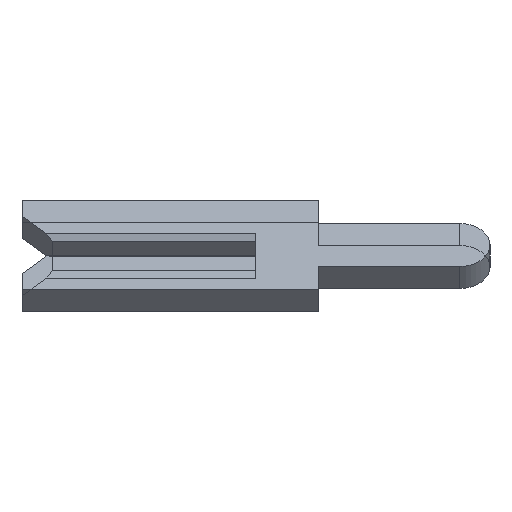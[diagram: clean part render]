
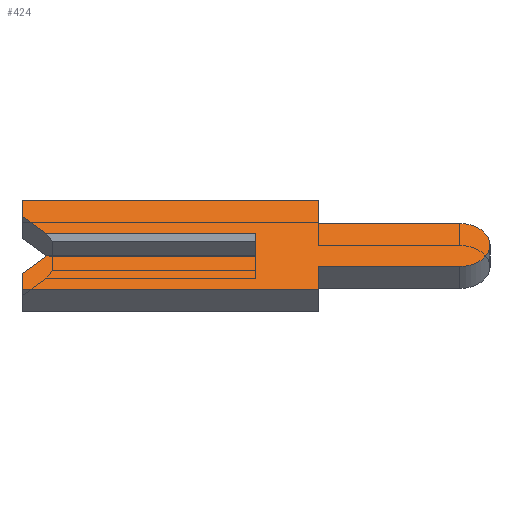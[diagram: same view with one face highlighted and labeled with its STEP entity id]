
A CAD part, left-side view. The second image highlights one B-rep face of the part: STEP entity #424.
In plain terms, the highlighted face is planar.
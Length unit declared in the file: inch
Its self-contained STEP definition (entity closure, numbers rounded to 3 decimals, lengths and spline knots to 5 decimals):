
#23 = CARTESIAN_POINT ( 'NONE',  ( -0.01, 0.15, -0.04 ) ) ;
#83 = EDGE_CURVE ( 'NONE', #255, #358, #2356, .T. ) ;
#101 = DIRECTION ( 'NONE',  ( 0., -0.707, 0.707 ) ) ;
#140 = CARTESIAN_POINT ( 'NONE',  ( -0.01, 0.15, 0.026 ) ) ;
#164 = ORIENTED_EDGE ( 'NONE', *, *, #291, .F. ) ;
#168 = VERTEX_POINT ( 'NONE', #1478 ) ;
#182 = CARTESIAN_POINT ( 'NONE',  ( -0.01, -0.1305, 0. ) ) ;
#186 = ORIENTED_EDGE ( 'NONE', *, *, #1485, .F. ) ;
#209 = DIRECTION ( 'NONE',  ( 1., 0., 0. ) ) ;
#237 = CARTESIAN_POINT ( 'NONE',  ( -0.01, -0.04, 0.04 ) ) ;
#255 = VERTEX_POINT ( 'NONE', #1156 ) ;
#263 = ORIENTED_EDGE ( 'NONE', *, *, #1547, .F. ) ;
#282 = LINE ( 'NONE', #1671, #1463 ) ;
#291 = EDGE_CURVE ( 'NONE', #1803, #767, #359, .T. ) ;
#296 = CARTESIAN_POINT ( 'NONE',  ( -0.01, 0.15, -0.04 ) ) ;
#314 = CARTESIAN_POINT ( 'NONE',  ( -0.01, -0.04, -0.04 ) ) ;
#356 = CARTESIAN_POINT ( 'NONE',  ( -0.01, 0.134, 0.01 ) ) ;
#358 = VERTEX_POINT ( 'NONE', #792 ) ;
#359 = CIRCLE ( 'NONE', #2261, 0.0195 ) ;
#362 = DIRECTION ( 'NONE',  ( 0., 0., -1. ) ) ;
#392 = VERTEX_POINT ( 'NONE', #2096 ) ;
#398 = LINE ( 'NONE', #314, #453 ) ;
#424 = ADVANCED_FACE ( 'NONE', ( #522 ), #2072, .F. ) ;
#453 = VECTOR ( 'NONE', #362, 39.37008 ) ;
#460 = VECTOR ( 'NONE', #2363, 39.37008 ) ;
#462 = EDGE_CURVE ( 'NONE', #1293, #1541, #1166, .T. ) ;
#512 = ORIENTED_EDGE ( 'NONE', *, *, #982, .F. ) ;
#518 = DIRECTION ( 'NONE',  ( 0., -1., 0. ) ) ;
#522 = FACE_OUTER_BOUND ( 'NONE', #2116, .T. ) ;
#554 = LINE ( 'NONE', #2094, #1105 ) ;
#566 = ORIENTED_EDGE ( 'NONE', *, *, #1073, .F. ) ;
#576 = VERTEX_POINT ( 'NONE', #1720 ) ;
#665 = ORIENTED_EDGE ( 'NONE', *, *, #1160, .F. ) ;
#724 = DIRECTION ( 'NONE',  ( 0., 1., 0. ) ) ;
#741 = CARTESIAN_POINT ( 'NONE',  ( -0.01, 0.1305, -0.0065 ) ) ;
#767 = VERTEX_POINT ( 'NONE', #2306 ) ;
#768 = VERTEX_POINT ( 'NONE', #832 ) ;
#772 = EDGE_CURVE ( 'NONE', #2245, #2060, #1546, .T. ) ;
#792 = CARTESIAN_POINT ( 'NONE',  ( -0.01, 0.15, 0.04 ) ) ;
#796 = LINE ( 'NONE', #1836, #2134 ) ;
#832 = CARTESIAN_POINT ( 'NONE',  ( -0.01, 0.134, -0.01 ) ) ;
#917 = LINE ( 'NONE', #1814, #1806 ) ;
#949 = DIRECTION ( 'NONE',  ( 1., 0., 0. ) ) ;
#974 = LINE ( 'NONE', #1981, #460 ) ;
#982 = EDGE_CURVE ( 'NONE', #1633, #255, #974, .T. ) ;
#1001 = ORIENTED_EDGE ( 'NONE', *, *, #1575, .F. ) ;
#1003 = ORIENTED_EDGE ( 'NONE', *, *, #83, .F. ) ;
#1009 = ORIENTED_EDGE ( 'NONE', *, *, #1917, .F. ) ;
#1019 = LINE ( 'NONE', #1175, #1614 ) ;
#1044 = VECTOR ( 'NONE', #1359, 39.37008 ) ;
#1073 = EDGE_CURVE ( 'NONE', #2060, #1803, #917, .T. ) ;
#1084 = VECTOR ( 'NONE', #101, 39.37008 ) ;
#1097 = DIRECTION ( 'NONE',  ( 0., 0., 1. ) ) ;
#1105 = VECTOR ( 'NONE', #1532, 39.37008 ) ;
#1118 = ORIENTED_EDGE ( 'NONE', *, *, #462, .F. ) ;
#1153 = DIRECTION ( 'NONE',  ( 0., -1., 0. ) ) ;
#1156 = CARTESIAN_POINT ( 'NONE',  ( -0.01, 0.15, 0.026 ) ) ;
#1160 = EDGE_CURVE ( 'NONE', #768, #392, #1286, .T. ) ;
#1163 = ORIENTED_EDGE ( 'NONE', *, *, #2068, .F. ) ;
#1166 = LINE ( 'NONE', #23, #1044 ) ;
#1175 = CARTESIAN_POINT ( 'NONE',  ( -0.01, 0.15, 0.01 ) ) ;
#1286 = LINE ( 'NONE', #1444, #1367 ) ;
#1293 = VERTEX_POINT ( 'NONE', #2011 ) ;
#1346 = AXIS2_PLACEMENT_3D ( 'NONE', #1535, #209, #1550 ) ;
#1359 = DIRECTION ( 'NONE',  ( 0., 1., 0. ) ) ;
#1367 = VECTOR ( 'NONE', #518, 39.37008 ) ;
#1372 = DIRECTION ( 'NONE',  ( 0., 0., -1. ) ) ;
#1444 = CARTESIAN_POINT ( 'NONE',  ( -0.01, -0.1305, -0.01 ) ) ;
#1454 = VERTEX_POINT ( 'NONE', #2392 ) ;
#1463 = VECTOR ( 'NONE', #1097, 39.37008 ) ;
#1478 = CARTESIAN_POINT ( 'NONE',  ( -0.01, -0.04, -0.0195 ) ) ;
#1485 = EDGE_CURVE ( 'NONE', #392, #1454, #282, .T. ) ;
#1532 = DIRECTION ( 'NONE',  ( 0., 0., 1. ) ) ;
#1535 = CARTESIAN_POINT ( 'NONE',  ( -0.01, -0.1305, 0. ) ) ;
#1541 = VERTEX_POINT ( 'NONE', #296 ) ;
#1543 = CARTESIAN_POINT ( 'NONE',  ( -0.01, -0.04, 0.0195 ) ) ;
#1546 = LINE ( 'NONE', #237, #1690 ) ;
#1547 = EDGE_CURVE ( 'NONE', #168, #1293, #398, .T. ) ;
#1550 = DIRECTION ( 'NONE',  ( 0., 0., -1. ) ) ;
#1559 = VECTOR ( 'NONE', #1153, 39.37008 ) ;
#1575 = EDGE_CURVE ( 'NONE', #767, #168, #796, .T. ) ;
#1614 = VECTOR ( 'NONE', #1747, 39.37008 ) ;
#1627 = ORIENTED_EDGE ( 'NONE', *, *, #772, .F. ) ;
#1633 = VERTEX_POINT ( 'NONE', #356 ) ;
#1671 = CARTESIAN_POINT ( 'NONE',  ( -0.01, 0., 0.0065 ) ) ;
#1690 = VECTOR ( 'NONE', #1372, 39.37008 ) ;
#1720 = CARTESIAN_POINT ( 'NONE',  ( -0.01, 0.15, -0.026 ) ) ;
#1747 = DIRECTION ( 'NONE',  ( 0., -1., 0. ) ) ;
#1803 = VERTEX_POINT ( 'NONE', #1862 ) ;
#1806 = VECTOR ( 'NONE', #2370, 39.37008 ) ;
#1814 = CARTESIAN_POINT ( 'NONE',  ( -0.01, -0.04, 0.0195 ) ) ;
#1836 = CARTESIAN_POINT ( 'NONE',  ( -0.01, -0.04, -0.0195 ) ) ;
#1862 = CARTESIAN_POINT ( 'NONE',  ( -0.01, -0.1305, 0.0195 ) ) ;
#1904 = EDGE_CURVE ( 'NONE', #576, #768, #2104, .T. ) ;
#1917 = EDGE_CURVE ( 'NONE', #358, #2245, #2249, .T. ) ;
#1981 = CARTESIAN_POINT ( 'NONE',  ( -0.01, 0.1305, 0.0065 ) ) ;
#2011 = CARTESIAN_POINT ( 'NONE',  ( -0.01, -0.04, -0.04 ) ) ;
#2031 = ORIENTED_EDGE ( 'NONE', *, *, #2375, .T. ) ;
#2060 = VERTEX_POINT ( 'NONE', #1543 ) ;
#2068 = EDGE_CURVE ( 'NONE', #1541, #576, #554, .T. ) ;
#2069 = CARTESIAN_POINT ( 'NONE',  ( -0.01, 0.15, 0.04 ) ) ;
#2072 = PLANE ( 'NONE',  #1346 ) ;
#2080 = DIRECTION ( 'NONE',  ( 0., 0., -1. ) ) ;
#2089 = CARTESIAN_POINT ( 'NONE',  ( -0.01, -0.04, 0.04 ) ) ;
#2094 = CARTESIAN_POINT ( 'NONE',  ( -0.01, 0.15, -0.026 ) ) ;
#2096 = CARTESIAN_POINT ( 'NONE',  ( -0.01, 0., -0.01 ) ) ;
#2104 = LINE ( 'NONE', #741, #1084 ) ;
#2116 = EDGE_LOOP ( 'NONE', ( #2031, #186, #665, #2148, #1163, #1118, #263, #1001, #164, #566, #1627, #1009, #1003, #512 ) ) ;
#2134 = VECTOR ( 'NONE', #724, 39.37008 ) ;
#2148 = ORIENTED_EDGE ( 'NONE', *, *, #1904, .F. ) ;
#2231 = DIRECTION ( 'NONE',  ( 0., 0., 1. ) ) ;
#2245 = VERTEX_POINT ( 'NONE', #2089 ) ;
#2249 = LINE ( 'NONE', #2069, #1559 ) ;
#2261 = AXIS2_PLACEMENT_3D ( 'NONE', #182, #949, #2080 ) ;
#2292 = VECTOR ( 'NONE', #2231, 39.37008 ) ;
#2306 = CARTESIAN_POINT ( 'NONE',  ( -0.01, -0.1305, -0.0195 ) ) ;
#2356 = LINE ( 'NONE', #140, #2292 ) ;
#2363 = DIRECTION ( 'NONE',  ( 0., 0.707, 0.707 ) ) ;
#2370 = DIRECTION ( 'NONE',  ( 0., -1., 0. ) ) ;
#2375 = EDGE_CURVE ( 'NONE', #1633, #1454, #1019, .T. ) ;
#2392 = CARTESIAN_POINT ( 'NONE',  ( -0.01, 0., 0.01 ) ) ;
